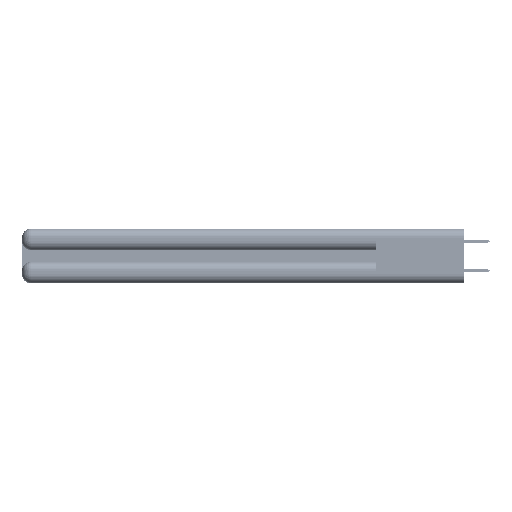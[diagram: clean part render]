
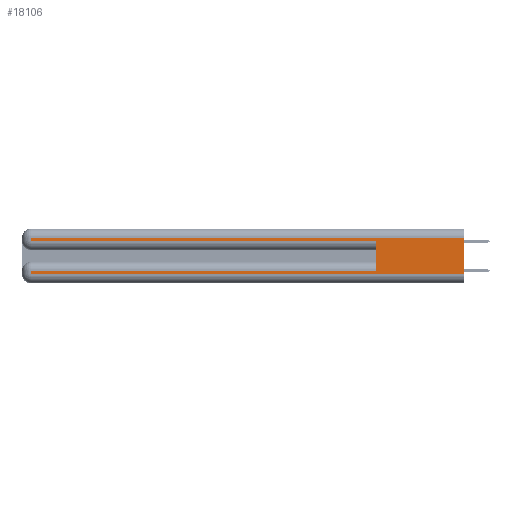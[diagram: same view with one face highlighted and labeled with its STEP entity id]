
A CAD part, left-side view. The second image highlights one B-rep face of the part: STEP entity #18106.
In plain terms, the highlighted planar face has unit normal (-1, 0, 0).
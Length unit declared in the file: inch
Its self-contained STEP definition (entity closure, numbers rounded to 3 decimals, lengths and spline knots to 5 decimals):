
#86 = VERTEX_POINT ( 'NONE', #17357 ) ;
#285 = LINE ( 'NONE', #29650, #41405 ) ;
#2946 = EDGE_CURVE ( 'NONE', #21063, #30007, #9211, .T. ) ;
#3608 = ORIENTED_EDGE ( 'NONE', *, *, #25750, .T. ) ;
#5328 = CARTESIAN_POINT ( 'NONE',  ( 0., 0., 0.06 ) ) ;
#5372 = PLANE ( 'NONE',  #17819 ) ;
#5444 = EDGE_LOOP ( 'NONE', ( #28568, #40971, #3608, #25531, #8021, #9985, #13743, #44730 ) ) ;
#6457 = CARTESIAN_POINT ( 'NONE',  ( 0., 2.94, 0.06 ) ) ;
#6981 = LINE ( 'NONE', #7719, #47865 ) ;
#7006 = EDGE_CURVE ( 'NONE', #22927, #18894, #6981, .T. ) ;
#7719 = CARTESIAN_POINT ( 'NONE',  ( 0., 0., 0.285 ) ) ;
#7761 = CARTESIAN_POINT ( 'NONE',  ( 0., 2.94, 0.31 ) ) ;
#8021 = ORIENTED_EDGE ( 'NONE', *, *, #46190, .F. ) ;
#9211 = LINE ( 'NONE', #34111, #16047 ) ;
#9443 = DIRECTION ( 'NONE',  ( 1., 0., 0. ) ) ;
#9985 = ORIENTED_EDGE ( 'NONE', *, *, #33034, .T. ) ;
#10229 = FACE_OUTER_BOUND ( 'NONE', #5444, .T. ) ;
#11550 = DIRECTION ( 'NONE',  ( 0., 0., -1. ) ) ;
#12051 = CARTESIAN_POINT ( 'NONE',  ( 0., 0., 0.31 ) ) ;
#12104 = CARTESIAN_POINT ( 'NONE',  ( 0., 0., 0.085 ) ) ;
#13142 = LINE ( 'NONE', #23951, #33018 ) ;
#13290 = VECTOR ( 'NONE', #11550, 39.37008 ) ;
#13743 = ORIENTED_EDGE ( 'NONE', *, *, #24384, .T. ) ;
#14324 = DIRECTION ( 'NONE',  ( 0., -1., 0. ) ) ;
#14665 = CARTESIAN_POINT ( 'NONE',  ( 0., 0., 0.37 ) ) ;
#15080 = VERTEX_POINT ( 'NONE', #37306 ) ;
#15785 = DIRECTION ( 'NONE',  ( 0., -1., 0. ) ) ;
#16047 = VECTOR ( 'NONE', #14324, 39.37008 ) ;
#16833 = CARTESIAN_POINT ( 'NONE',  ( 0., 0.6, 0.285 ) ) ;
#17357 = CARTESIAN_POINT ( 'NONE',  ( 0., 2.94, 0.085 ) ) ;
#17819 = AXIS2_PLACEMENT_3D ( 'NONE', #48819, #9443, #37218 ) ;
#18089 = VECTOR ( 'NONE', #39154, 39.37008 ) ;
#18106 = ADVANCED_FACE ( 'NONE', ( #10229 ), #5372, .F. ) ;
#18630 = DIRECTION ( 'NONE',  ( 0., 0., -1. ) ) ;
#18894 = VERTEX_POINT ( 'NONE', #16833 ) ;
#19882 = VECTOR ( 'NONE', #18630, 39.37008 ) ;
#21063 = VERTEX_POINT ( 'NONE', #6457 ) ;
#22927 = VERTEX_POINT ( 'NONE', #37541 ) ;
#23951 = CARTESIAN_POINT ( 'NONE',  ( 0., 2.94, 0.37 ) ) ;
#24384 = EDGE_CURVE ( 'NONE', #86, #21063, #44859, .T. ) ;
#24437 = LINE ( 'NONE', #12051, #33740 ) ;
#25531 = ORIENTED_EDGE ( 'NONE', *, *, #7006, .T. ) ;
#25750 = EDGE_CURVE ( 'NONE', #39242, #22927, #13142, .T. ) ;
#28568 = ORIENTED_EDGE ( 'NONE', *, *, #50792, .F. ) ;
#29650 = CARTESIAN_POINT ( 'NONE',  ( 0., 0.6, 0.145 ) ) ;
#30007 = VERTEX_POINT ( 'NONE', #5328 ) ;
#33018 = VECTOR ( 'NONE', #43639, 39.37008 ) ;
#33034 = EDGE_CURVE ( 'NONE', #15080, #86, #48342, .T. ) ;
#33740 = VECTOR ( 'NONE', #39766, 39.37008 ) ;
#34111 = CARTESIAN_POINT ( 'NONE',  ( 0., 0., 0.06 ) ) ;
#37218 = DIRECTION ( 'NONE',  ( 0., 0., -1. ) ) ;
#37306 = CARTESIAN_POINT ( 'NONE',  ( 0., 0.6, 0.085 ) ) ;
#37439 = DIRECTION ( 'NONE',  ( 0., 0., 1. ) ) ;
#37541 = CARTESIAN_POINT ( 'NONE',  ( 0., 2.94, 0.285 ) ) ;
#39154 = DIRECTION ( 'NONE',  ( 0., 1., 0. ) ) ;
#39242 = VERTEX_POINT ( 'NONE', #7761 ) ;
#39277 = CARTESIAN_POINT ( 'NONE',  ( 0., 2.94, 0.37 ) ) ;
#39766 = DIRECTION ( 'NONE',  ( 0., 1., 0. ) ) ;
#40971 = ORIENTED_EDGE ( 'NONE', *, *, #49153, .T. ) ;
#41405 = VECTOR ( 'NONE', #37439, 39.37008 ) ;
#42993 = VERTEX_POINT ( 'NONE', #45806 ) ;
#43639 = DIRECTION ( 'NONE',  ( 0., 0., -1. ) ) ;
#44730 = ORIENTED_EDGE ( 'NONE', *, *, #2946, .T. ) ;
#44859 = LINE ( 'NONE', #39277, #13290 ) ;
#45806 = CARTESIAN_POINT ( 'NONE',  ( 0., 0., 0.31 ) ) ;
#46190 = EDGE_CURVE ( 'NONE', #15080, #18894, #285, .T. ) ;
#47865 = VECTOR ( 'NONE', #15785, 39.37008 ) ;
#48342 = LINE ( 'NONE', #12104, #18089 ) ;
#48819 = CARTESIAN_POINT ( 'NONE',  ( 0., 0., 0.37 ) ) ;
#49153 = EDGE_CURVE ( 'NONE', #42993, #39242, #24437, .T. ) ;
#50792 = EDGE_CURVE ( 'NONE', #42993, #30007, #51266, .T. ) ;
#51266 = LINE ( 'NONE', #14665, #19882 ) ;
